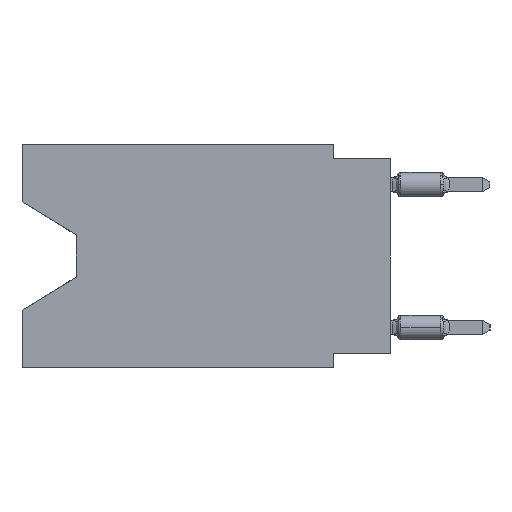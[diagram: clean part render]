
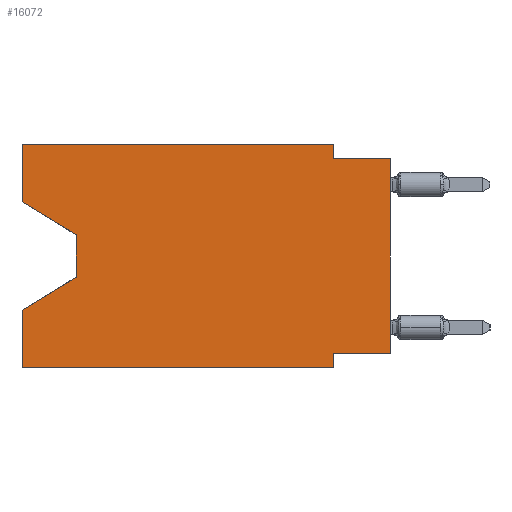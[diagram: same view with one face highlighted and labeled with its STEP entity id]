
A CAD part, left-side view. The second image highlights one B-rep face of the part: STEP entity #16072.
In plain terms, the highlighted planar face has unit normal (-1, 0, 0).
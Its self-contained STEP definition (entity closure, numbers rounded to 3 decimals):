
#255 = DIRECTION ( 'NONE',  ( 0., 0., 1. ) ) ;
#493 = LINE ( 'NONE', #4409, #10166 ) ;
#928 = LINE ( 'NONE', #8390, #12202 ) ;
#1794 = ORIENTED_EDGE ( 'NONE', *, *, #11250, .F. ) ;
#1835 = CARTESIAN_POINT ( 'NONE',  ( 0., 16.383, -7.36 ) ) ;
#2042 = CARTESIAN_POINT ( 'NONE',  ( 0., 2.54, -9.906 ) ) ;
#2052 = DIRECTION ( 'NONE',  ( 0., -0.855, -0.519 ) ) ;
#2104 = DIRECTION ( 'NONE',  ( 0., 0., -1. ) ) ;
#2264 = EDGE_CURVE ( 'NONE', #12885, #4231, #493, .T. ) ;
#2457 = LINE ( 'NONE', #18993, #22023 ) ;
#2537 = DIRECTION ( 'NONE',  ( 0., 1., 0. ) ) ;
#2987 = ORIENTED_EDGE ( 'NONE', *, *, #10740, .F. ) ;
#3028 = ORIENTED_EDGE ( 'NONE', *, *, #22373, .F. ) ;
#3377 = VECTOR ( 'NONE', #7785, 1000. ) ;
#3403 = LINE ( 'NONE', #10624, #14150 ) ;
#3699 = VERTEX_POINT ( 'NONE', #1835 ) ;
#3935 = CARTESIAN_POINT ( 'NONE',  ( 0., 16.383, 0. ) ) ;
#4004 = LINE ( 'NONE', #14780, #21219 ) ;
#4231 = VERTEX_POINT ( 'NONE', #2042 ) ;
#4409 = CARTESIAN_POINT ( 'NONE',  ( 0., 16.383, -9.906 ) ) ;
#5233 = VECTOR ( 'NONE', #19914, 1000. ) ;
#5821 = ORIENTED_EDGE ( 'NONE', *, *, #17512, .F. ) ;
#5822 = CARTESIAN_POINT ( 'NONE',  ( 0., 0., -0.635 ) ) ;
#5996 = VECTOR ( 'NONE', #255, 1000. ) ;
#6124 = DIRECTION ( 'NONE',  ( 0., -1., 0. ) ) ;
#6258 = EDGE_CURVE ( 'NONE', #23281, #10722, #18938, .T. ) ;
#6923 = VERTEX_POINT ( 'NONE', #20220 ) ;
#6963 = VECTOR ( 'NONE', #12676, 1000. ) ;
#6990 = EDGE_CURVE ( 'NONE', #19051, #6923, #10889, .T. ) ;
#7190 = ORIENTED_EDGE ( 'NONE', *, *, #20045, .F. ) ;
#7260 = PLANE ( 'NONE',  #17697 ) ;
#7701 = CARTESIAN_POINT ( 'NONE',  ( 0., 16.383, 0. ) ) ;
#7785 = DIRECTION ( 'NONE',  ( 0., 0., -1. ) ) ;
#7967 = CARTESIAN_POINT ( 'NONE',  ( 0., 13.97, -5.893 ) ) ;
#8390 = CARTESIAN_POINT ( 'NONE',  ( 0., 0., -9.271 ) ) ;
#8727 = VECTOR ( 'NONE', #16517, 1000. ) ;
#8995 = CARTESIAN_POINT ( 'NONE',  ( 0., 0., 0. ) ) ;
#9011 = EDGE_CURVE ( 'NONE', #9446, #9820, #10834, .T. ) ;
#9446 = VERTEX_POINT ( 'NONE', #20443 ) ;
#9734 = CARTESIAN_POINT ( 'NONE',  ( 0., 13.97, -4.013 ) ) ;
#9820 = VERTEX_POINT ( 'NONE', #5822 ) ;
#10166 = VECTOR ( 'NONE', #11874, 1000. ) ;
#10202 = ORIENTED_EDGE ( 'NONE', *, *, #6258, .T. ) ;
#10624 = CARTESIAN_POINT ( 'NONE',  ( 0., 13.97, -5.893 ) ) ;
#10722 = VERTEX_POINT ( 'NONE', #7967 ) ;
#10740 = EDGE_CURVE ( 'NONE', #6923, #23727, #2457, .T. ) ;
#10834 = LINE ( 'NONE', #8995, #6963 ) ;
#10889 = LINE ( 'NONE', #7701, #12051 ) ;
#11085 = ORIENTED_EDGE ( 'NONE', *, *, #22022, .T. ) ;
#11250 = EDGE_CURVE ( 'NONE', #19760, #4231, #16479, .T. ) ;
#11392 = EDGE_LOOP ( 'NONE', ( #19461, #10202, #11085, #13995, #19056, #1794, #3028, #23800, #7190, #5821, #2987, #16346 ) ) ;
#11399 = DIRECTION ( 'NONE',  ( 1., 0., 0. ) ) ;
#11874 = DIRECTION ( 'NONE',  ( 0., -1., 0. ) ) ;
#12051 = VECTOR ( 'NONE', #18367, 1000. ) ;
#12202 = VECTOR ( 'NONE', #2537, 1000. ) ;
#12676 = DIRECTION ( 'NONE',  ( 0., 0., 1. ) ) ;
#12683 = CARTESIAN_POINT ( 'NONE',  ( 0., 2.54, 0. ) ) ;
#12824 = LINE ( 'NONE', #22011, #8727 ) ;
#12885 = VERTEX_POINT ( 'NONE', #17474 ) ;
#13486 = CARTESIAN_POINT ( 'NONE',  ( 0., 2.54, -9.271 ) ) ;
#13995 = ORIENTED_EDGE ( 'NONE', *, *, #23027, .F. ) ;
#14150 = VECTOR ( 'NONE', #20077, 1000. ) ;
#14780 = CARTESIAN_POINT ( 'NONE',  ( 0., 16.383, -2.546 ) ) ;
#15880 = CARTESIAN_POINT ( 'NONE',  ( 0., 16.383, -2.546 ) ) ;
#16072 = ADVANCED_FACE ( 'NONE', ( #20248 ), #7260, .F. ) ;
#16103 = CARTESIAN_POINT ( 'NONE',  ( 0., 2.54, -9.906 ) ) ;
#16346 = ORIENTED_EDGE ( 'NONE', *, *, #6990, .F. ) ;
#16479 = LINE ( 'NONE', #16103, #5233 ) ;
#16517 = DIRECTION ( 'NONE',  ( 0., 0., -1. ) ) ;
#17030 = LINE ( 'NONE', #22523, #5996 ) ;
#17275 = CARTESIAN_POINT ( 'NONE',  ( 0., 0., -0.635 ) ) ;
#17474 = CARTESIAN_POINT ( 'NONE',  ( 0., 16.383, -9.906 ) ) ;
#17512 = EDGE_CURVE ( 'NONE', #23727, #21152, #12824, .T. ) ;
#17697 = AXIS2_PLACEMENT_3D ( 'NONE', #3935, #11399, #2104 ) ;
#17804 = CARTESIAN_POINT ( 'NONE',  ( 0., 2.54, -0.635 ) ) ;
#18367 = DIRECTION ( 'NONE',  ( 0., 0., 1. ) ) ;
#18938 = LINE ( 'NONE', #9734, #3377 ) ;
#18993 = CARTESIAN_POINT ( 'NONE',  ( 0., 16.383, 0. ) ) ;
#19051 = VERTEX_POINT ( 'NONE', #15880 ) ;
#19056 = ORIENTED_EDGE ( 'NONE', *, *, #2264, .T. ) ;
#19363 = VECTOR ( 'NONE', #6124, 1000. ) ;
#19461 = ORIENTED_EDGE ( 'NONE', *, *, #22196, .T. ) ;
#19760 = VERTEX_POINT ( 'NONE', #13486 ) ;
#19914 = DIRECTION ( 'NONE',  ( 0., 0., -1. ) ) ;
#20045 = EDGE_CURVE ( 'NONE', #21152, #9820, #20948, .T. ) ;
#20077 = DIRECTION ( 'NONE',  ( 0., 0.855, -0.519 ) ) ;
#20220 = CARTESIAN_POINT ( 'NONE',  ( 0., 16.383, 0. ) ) ;
#20248 = FACE_OUTER_BOUND ( 'NONE', #11392, .T. ) ;
#20443 = CARTESIAN_POINT ( 'NONE',  ( 0., 0., -9.271 ) ) ;
#20948 = LINE ( 'NONE', #17275, #19363 ) ;
#21152 = VERTEX_POINT ( 'NONE', #17804 ) ;
#21197 = DIRECTION ( 'NONE',  ( 0., -1., 0. ) ) ;
#21219 = VECTOR ( 'NONE', #2052, 1000. ) ;
#21773 = CARTESIAN_POINT ( 'NONE',  ( 0., 13.97, -4.013 ) ) ;
#22011 = CARTESIAN_POINT ( 'NONE',  ( 0., 2.54, 0. ) ) ;
#22022 = EDGE_CURVE ( 'NONE', #10722, #3699, #3403, .T. ) ;
#22023 = VECTOR ( 'NONE', #21197, 1000. ) ;
#22196 = EDGE_CURVE ( 'NONE', #19051, #23281, #4004, .T. ) ;
#22373 = EDGE_CURVE ( 'NONE', #9446, #19760, #928, .T. ) ;
#22523 = CARTESIAN_POINT ( 'NONE',  ( 0., 16.383, 0. ) ) ;
#23027 = EDGE_CURVE ( 'NONE', #12885, #3699, #17030, .T. ) ;
#23281 = VERTEX_POINT ( 'NONE', #21773 ) ;
#23727 = VERTEX_POINT ( 'NONE', #12683 ) ;
#23800 = ORIENTED_EDGE ( 'NONE', *, *, #9011, .T. ) ;
